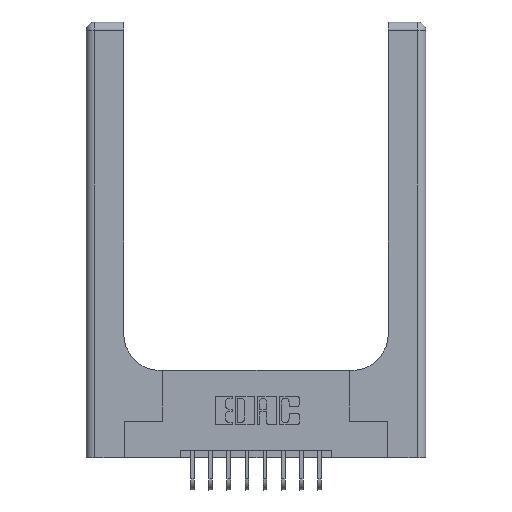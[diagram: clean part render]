
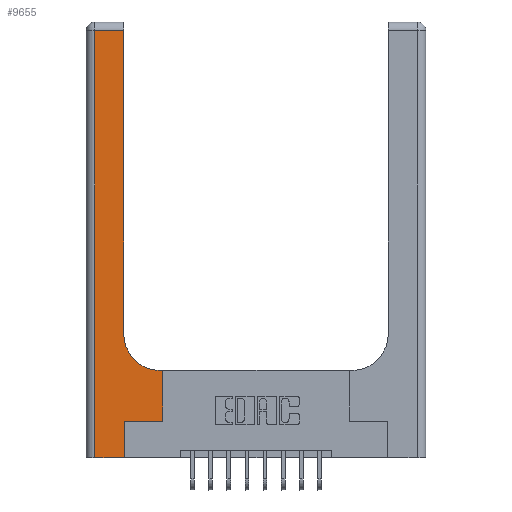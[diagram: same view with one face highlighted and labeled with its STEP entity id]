
A CAD part, top view. The second image highlights one B-rep face of the part: STEP entity #9655.
In plain terms, the highlighted planar face has unit normal (0, 0, 1).
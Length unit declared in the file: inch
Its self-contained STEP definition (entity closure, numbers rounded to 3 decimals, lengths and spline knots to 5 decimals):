
#15 = DIRECTION ( 'NONE',  ( -1., 0., 0. ) ) ;
#28 = VERTEX_POINT ( 'NONE', #5990 ) ;
#280 = VECTOR ( 'NONE', #17176, 39.37008 ) ;
#614 = EDGE_CURVE ( 'NONE', #10555, #2751, #4055, .T. ) ;
#703 = DIRECTION ( 'NONE',  ( 0., 1., 0. ) ) ;
#949 = EDGE_CURVE ( 'NONE', #2751, #1669, #2965, .T. ) ;
#1007 = EDGE_CURVE ( 'NONE', #13390, #12242, #5901, .T. ) ;
#1053 = LINE ( 'NONE', #1138, #5088 ) ;
#1138 = CARTESIAN_POINT ( 'NONE',  ( 0.26, 3., 0.37 ) ) ;
#1351 = CIRCLE ( 'NONE', #4959, 0.25 ) ;
#1466 = CARTESIAN_POINT ( 'NONE',  ( 0.26, 0.85, 0.37 ) ) ;
#1538 = DIRECTION ( 'NONE',  ( -1., 0., 0. ) ) ;
#1616 = CARTESIAN_POINT ( 'NONE',  ( 0.51, 0.85, 0.37 ) ) ;
#1669 = VERTEX_POINT ( 'NONE', #13530 ) ;
#1726 = DIRECTION ( 'NONE',  ( 1., 0., 0. ) ) ;
#1842 = ORIENTED_EDGE ( 'NONE', *, *, #13487, .T. ) ;
#2751 = VERTEX_POINT ( 'NONE', #7615 ) ;
#2965 = LINE ( 'NONE', #8335, #6832 ) ;
#3105 = ORIENTED_EDGE ( 'NONE', *, *, #614, .T. ) ;
#3194 = CARTESIAN_POINT ( 'NONE',  ( 0.265, 0., 0.37 ) ) ;
#4023 = LINE ( 'NONE', #5326, #280 ) ;
#4055 = LINE ( 'NONE', #16467, #8504 ) ;
#4149 = DIRECTION ( 'NONE',  ( 1., 0., 0. ) ) ;
#4259 = DIRECTION ( 'NONE',  ( -1., 0., 0. ) ) ;
#4490 = VECTOR ( 'NONE', #15, 39.37008 ) ;
#4623 = VECTOR ( 'NONE', #15147, 39.37008 ) ;
#4959 = AXIS2_PLACEMENT_3D ( 'NONE', #1616, #6996, #4149 ) ;
#5088 = VECTOR ( 'NONE', #6361, 39.37008 ) ;
#5295 = CARTESIAN_POINT ( 'NONE',  ( 0.26, 2.94, 0.37 ) ) ;
#5326 = CARTESIAN_POINT ( 'NONE',  ( 0.528, 0.25, 0.37 ) ) ;
#5901 = LINE ( 'NONE', #9737, #4623 ) ;
#5990 = CARTESIAN_POINT ( 'NONE',  ( 0.51, 0.6, 0.37 ) ) ;
#6361 = DIRECTION ( 'NONE',  ( 0., 1., 0. ) ) ;
#6685 = ORIENTED_EDGE ( 'NONE', *, *, #11639, .T. ) ;
#6832 = VECTOR ( 'NONE', #1726, 39.37008 ) ;
#6996 = DIRECTION ( 'NONE',  ( 0., 0., -1. ) ) ;
#7118 = CARTESIAN_POINT ( 'NONE',  ( 0.528, 0.6, 0.37 ) ) ;
#7364 = VERTEX_POINT ( 'NONE', #1466 ) ;
#7615 = CARTESIAN_POINT ( 'NONE',  ( 0.265, 0.25, 0.37 ) ) ;
#7648 = ORIENTED_EDGE ( 'NONE', *, *, #14722, .T. ) ;
#7770 = ORIENTED_EDGE ( 'NONE', *, *, #1007, .T. ) ;
#7845 = EDGE_CURVE ( 'NONE', #8671, #28, #13454, .T. ) ;
#7984 = EDGE_CURVE ( 'NONE', #1669, #8671, #4023, .T. ) ;
#8335 = CARTESIAN_POINT ( 'NONE',  ( 0.265, 0.25, 0.37 ) ) ;
#8504 = VECTOR ( 'NONE', #703, 39.37008 ) ;
#8671 = VERTEX_POINT ( 'NONE', #7118 ) ;
#9655 = ADVANCED_FACE ( 'NONE', ( #13568 ), #9825, .F. ) ;
#9737 = CARTESIAN_POINT ( 'NONE',  ( 0.06, 3., 0.37 ) ) ;
#9825 = PLANE ( 'NONE',  #10098 ) ;
#9926 = VERTEX_POINT ( 'NONE', #5295 ) ;
#10098 = AXIS2_PLACEMENT_3D ( 'NONE', #16448, #13650, #4259 ) ;
#10555 = VERTEX_POINT ( 'NONE', #3194 ) ;
#10636 = ORIENTED_EDGE ( 'NONE', *, *, #7984, .T. ) ;
#10758 = CARTESIAN_POINT ( 'NONE',  ( 0.26, 0.6, 0.37 ) ) ;
#10796 = VECTOR ( 'NONE', #11426, 39.37008 ) ;
#11426 = DIRECTION ( 'NONE',  ( 1., 0., 0. ) ) ;
#11639 = EDGE_CURVE ( 'NONE', #28, #7364, #1351, .T. ) ;
#11741 = EDGE_LOOP ( 'NONE', ( #1842, #7648, #7770, #15753, #3105, #12139, #10636, #13946, #6685 ) ) ;
#11794 = EDGE_CURVE ( 'NONE', #12242, #10555, #15549, .T. ) ;
#12139 = ORIENTED_EDGE ( 'NONE', *, *, #949, .T. ) ;
#12174 = LINE ( 'NONE', #13328, #4490 ) ;
#12242 = VERTEX_POINT ( 'NONE', #17173 ) ;
#12974 = CARTESIAN_POINT ( 'NONE',  ( 0.06, 2.94, 0.37 ) ) ;
#13328 = CARTESIAN_POINT ( 'NONE',  ( 0., 2.94, 0.37 ) ) ;
#13390 = VERTEX_POINT ( 'NONE', #12974 ) ;
#13454 = LINE ( 'NONE', #10758, #16387 ) ;
#13487 = EDGE_CURVE ( 'NONE', #7364, #9926, #1053, .T. ) ;
#13530 = CARTESIAN_POINT ( 'NONE',  ( 0.528, 0.25, 0.37 ) ) ;
#13568 = FACE_OUTER_BOUND ( 'NONE', #11741, .T. ) ;
#13650 = DIRECTION ( 'NONE',  ( 0., 0., -1. ) ) ;
#13879 = CARTESIAN_POINT ( 'NONE',  ( 0., 0., 0.37 ) ) ;
#13946 = ORIENTED_EDGE ( 'NONE', *, *, #7845, .T. ) ;
#14722 = EDGE_CURVE ( 'NONE', #9926, #13390, #12174, .T. ) ;
#15147 = DIRECTION ( 'NONE',  ( 0., -1., 0. ) ) ;
#15549 = LINE ( 'NONE', #13879, #10796 ) ;
#15753 = ORIENTED_EDGE ( 'NONE', *, *, #11794, .T. ) ;
#16387 = VECTOR ( 'NONE', #1538, 39.37008 ) ;
#16448 = CARTESIAN_POINT ( 'NONE',  ( 0., 3., 0.37 ) ) ;
#16467 = CARTESIAN_POINT ( 'NONE',  ( 0.265, 0., 0.37 ) ) ;
#17173 = CARTESIAN_POINT ( 'NONE',  ( 0.06, 0., 0.37 ) ) ;
#17176 = DIRECTION ( 'NONE',  ( 0., 1., 0. ) ) ;
